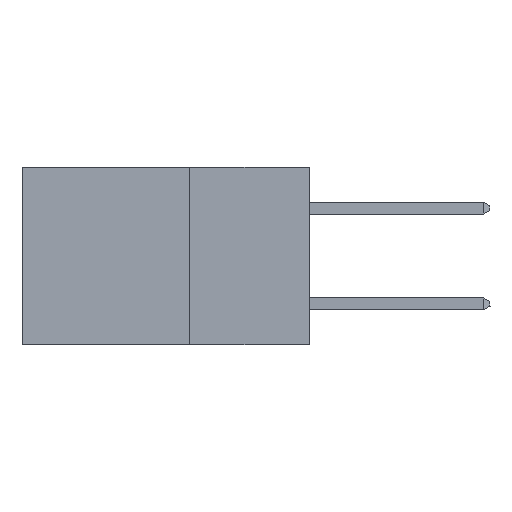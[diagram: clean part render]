
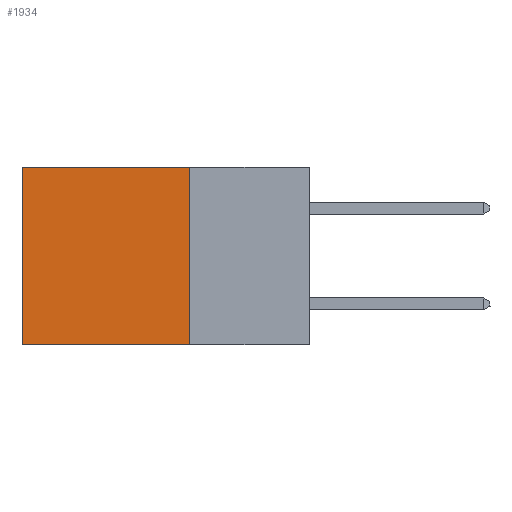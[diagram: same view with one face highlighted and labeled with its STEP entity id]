
A CAD part, left-side view. The second image highlights one B-rep face of the part: STEP entity #1934.
In plain terms, the highlighted planar face has unit normal (-1, 0, 0).
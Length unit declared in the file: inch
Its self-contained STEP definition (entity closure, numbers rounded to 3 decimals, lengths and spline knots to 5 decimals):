
#8 = CARTESIAN_POINT ( 'NONE',  ( 0.2875, 0.25, 0. ) ) ;
#1934 = ADVANCED_FACE ( 'NONE', ( #18087 ), #12805, .F. ) ;
#2216 = VECTOR ( 'NONE', #17552, 39.37008 ) ;
#2798 = LINE ( 'NONE', #17683, #25541 ) ;
#3815 = CARTESIAN_POINT ( 'NONE',  ( 0.2875, 0.25, 0. ) ) ;
#4260 = DIRECTION ( 'NONE',  ( 0., 0., -1. ) ) ;
#5410 = VERTEX_POINT ( 'NONE', #5636 ) ;
#5636 = CARTESIAN_POINT ( 'NONE',  ( 0.2875, 0.6, -0.37 ) ) ;
#6087 = VECTOR ( 'NONE', #15671, 39.37008 ) ;
#6454 = EDGE_LOOP ( 'NONE', ( #11411, #8710, #27832, #27348 ) ) ;
#6852 = CARTESIAN_POINT ( 'NONE',  ( 0.2875, 0.25, -0.37 ) ) ;
#7481 = AXIS2_PLACEMENT_3D ( 'NONE', #3815, #8507, #9175 ) ;
#7799 = CARTESIAN_POINT ( 'NONE',  ( 0.2875, 0.6, 0. ) ) ;
#8507 = DIRECTION ( 'NONE',  ( 1., 0., 0. ) ) ;
#8710 = ORIENTED_EDGE ( 'NONE', *, *, #28051, .F. ) ;
#8932 = LINE ( 'NONE', #28128, #2216 ) ;
#9175 = DIRECTION ( 'NONE',  ( 0., 0., -1. ) ) ;
#10614 = VECTOR ( 'NONE', #4260, 39.37008 ) ;
#10948 = EDGE_CURVE ( 'NONE', #17351, #19806, #27984, .T. ) ;
#11411 = ORIENTED_EDGE ( 'NONE', *, *, #18773, .T. ) ;
#11662 = VERTEX_POINT ( 'NONE', #6852 ) ;
#12805 = PLANE ( 'NONE',  #7481 ) ;
#15402 = CARTESIAN_POINT ( 'NONE',  ( 0.2875, 0.25, 0. ) ) ;
#15671 = DIRECTION ( 'NONE',  ( 0., 1., 0. ) ) ;
#17351 = VERTEX_POINT ( 'NONE', #28014 ) ;
#17552 = DIRECTION ( 'NONE',  ( 0., 1., 0. ) ) ;
#17683 = CARTESIAN_POINT ( 'NONE',  ( 0.2875, 0.6, 0. ) ) ;
#18087 = FACE_OUTER_BOUND ( 'NONE', #6454, .T. ) ;
#18232 = EDGE_CURVE ( 'NONE', #17351, #11662, #22245, .T. ) ;
#18773 = EDGE_CURVE ( 'NONE', #19806, #5410, #2798, .T. ) ;
#19806 = VERTEX_POINT ( 'NONE', #7799 ) ;
#22245 = LINE ( 'NONE', #15402, #10614 ) ;
#24149 = DIRECTION ( 'NONE',  ( 0., 0., -1. ) ) ;
#25541 = VECTOR ( 'NONE', #24149, 39.37008 ) ;
#27348 = ORIENTED_EDGE ( 'NONE', *, *, #10948, .T. ) ;
#27832 = ORIENTED_EDGE ( 'NONE', *, *, #18232, .F. ) ;
#27984 = LINE ( 'NONE', #8, #6087 ) ;
#28014 = CARTESIAN_POINT ( 'NONE',  ( 0.2875, 0.25, 0. ) ) ;
#28051 = EDGE_CURVE ( 'NONE', #11662, #5410, #8932, .T. ) ;
#28128 = CARTESIAN_POINT ( 'NONE',  ( 0.2875, 0.25, -0.37 ) ) ;
